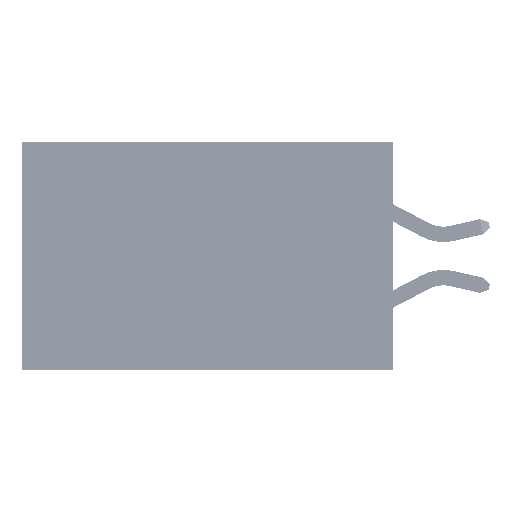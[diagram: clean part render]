
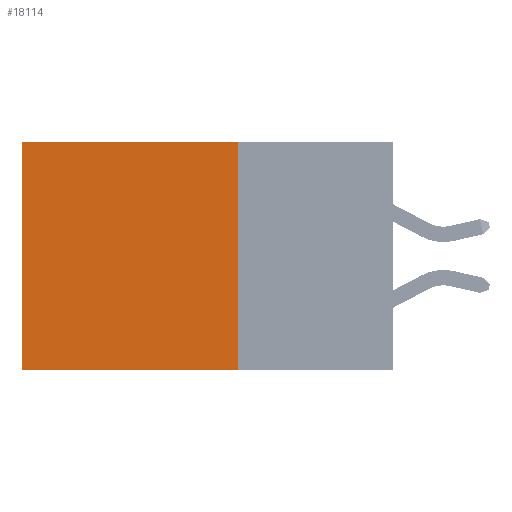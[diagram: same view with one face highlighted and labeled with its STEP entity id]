
A CAD part, left-side view. The second image highlights one B-rep face of the part: STEP entity #18114.
In plain terms, the highlighted planar face has unit normal (-1, 0, 0).
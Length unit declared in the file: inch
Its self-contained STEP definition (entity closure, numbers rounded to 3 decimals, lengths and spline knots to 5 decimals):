
#638 = LINE ( 'NONE', #9059, #38469 ) ;
#1211 = VECTOR ( 'NONE', #36862, 39.37008 ) ;
#4564 = EDGE_CURVE ( 'NONE', #36090, #20659, #638, .T. ) ;
#5700 = VECTOR ( 'NONE', #26327, 39.37008 ) ;
#6189 = AXIS2_PLACEMENT_3D ( 'NONE', #29189, #25532, #36604 ) ;
#7336 = VECTOR ( 'NONE', #34191, 39.37008 ) ;
#7840 = VERTEX_POINT ( 'NONE', #24586 ) ;
#9059 = CARTESIAN_POINT ( 'NONE',  ( 0.2875, 0.25, 0. ) ) ;
#9248 = EDGE_CURVE ( 'NONE', #20659, #34252, #44099, .T. ) ;
#15711 = ORIENTED_EDGE ( 'NONE', *, *, #4564, .F. ) ;
#18114 = ADVANCED_FACE ( 'NONE', ( #37953 ), #43348, .F. ) ;
#19893 = LINE ( 'NONE', #34340, #7336 ) ;
#20254 = EDGE_CURVE ( 'NONE', #7840, #34252, #19893, .T. ) ;
#20659 = VERTEX_POINT ( 'NONE', #40078 ) ;
#24586 = CARTESIAN_POINT ( 'NONE',  ( 0.2875, 0.6, 0. ) ) ;
#25532 = DIRECTION ( 'NONE',  ( 1., 0., 0. ) ) ;
#25680 = CARTESIAN_POINT ( 'NONE',  ( 0.2875, 0.25, 0. ) ) ;
#26327 = DIRECTION ( 'NONE',  ( 0., 1., 0. ) ) ;
#26994 = EDGE_CURVE ( 'NONE', #36090, #7840, #30410, .T. ) ;
#29189 = CARTESIAN_POINT ( 'NONE',  ( 0.2875, 0.25, 0. ) ) ;
#30410 = LINE ( 'NONE', #44085, #1211 ) ;
#34191 = DIRECTION ( 'NONE',  ( 0., 0., -1. ) ) ;
#34252 = VERTEX_POINT ( 'NONE', #37255 ) ;
#34340 = CARTESIAN_POINT ( 'NONE',  ( 0.2875, 0.6, 0. ) ) ;
#36090 = VERTEX_POINT ( 'NONE', #25680 ) ;
#36604 = DIRECTION ( 'NONE',  ( 0., 0., -1. ) ) ;
#36862 = DIRECTION ( 'NONE',  ( 0., 1., 0. ) ) ;
#37179 = ORIENTED_EDGE ( 'NONE', *, *, #20254, .T. ) ;
#37255 = CARTESIAN_POINT ( 'NONE',  ( 0.2875, 0.6, -0.37 ) ) ;
#37953 = FACE_OUTER_BOUND ( 'NONE', #45402, .T. ) ;
#38469 = VECTOR ( 'NONE', #42676, 39.37008 ) ;
#38894 = ORIENTED_EDGE ( 'NONE', *, *, #26994, .T. ) ;
#40078 = CARTESIAN_POINT ( 'NONE',  ( 0.2875, 0.25, -0.37 ) ) ;
#42120 = ORIENTED_EDGE ( 'NONE', *, *, #9248, .F. ) ;
#42676 = DIRECTION ( 'NONE',  ( 0., 0., -1. ) ) ;
#43348 = PLANE ( 'NONE',  #6189 ) ;
#43472 = CARTESIAN_POINT ( 'NONE',  ( 0.2875, 0.25, -0.37 ) ) ;
#44085 = CARTESIAN_POINT ( 'NONE',  ( 0.2875, 0.25, 0. ) ) ;
#44099 = LINE ( 'NONE', #43472, #5700 ) ;
#45402 = EDGE_LOOP ( 'NONE', ( #37179, #42120, #15711, #38894 ) ) ;
